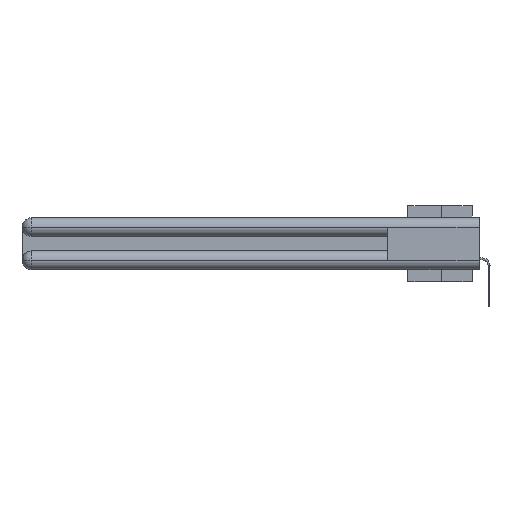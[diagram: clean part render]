
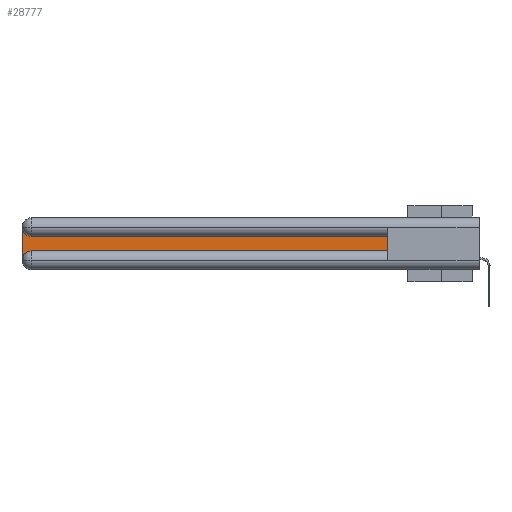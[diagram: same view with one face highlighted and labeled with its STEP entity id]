
A CAD part, left-side view. The second image highlights one B-rep face of the part: STEP entity #28777.
In plain terms, the highlighted planar face has unit normal (-1, 0, 0).
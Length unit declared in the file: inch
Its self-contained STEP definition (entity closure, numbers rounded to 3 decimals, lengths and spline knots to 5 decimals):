
#71 = DIRECTION ( 'NONE',  ( 0., 0., -1. ) ) ;
#74 = CARTESIAN_POINT ( 'NONE',  ( 0.075, 2.94, -0.2775 ) ) ;
#601 = AXIS2_PLACEMENT_3D ( 'NONE', #74, #2837, #3019 ) ;
#1091 = ORIENTED_EDGE ( 'NONE', *, *, #26982, .T. ) ;
#1092 = DIRECTION ( 'NONE',  ( 0., 0., -1. ) ) ;
#1126 = EDGE_CURVE ( 'NONE', #16371, #23580, #26672, .T. ) ;
#1837 = EDGE_CURVE ( 'NONE', #14054, #26302, #26580, .T. ) ;
#2837 = DIRECTION ( 'NONE',  ( 1., 0., 0. ) ) ;
#3019 = DIRECTION ( 'NONE',  ( 0., 0., -1. ) ) ;
#3077 = EDGE_CURVE ( 'NONE', #4866, #16371, #8599, .T. ) ;
#4682 = EDGE_CURVE ( 'NONE', #23580, #14054, #10926, .T. ) ;
#4866 = VERTEX_POINT ( 'NONE', #5899 ) ;
#5076 = CARTESIAN_POINT ( 'NONE',  ( 0.075, 0.6, -0.2175 ) ) ;
#5422 = FACE_OUTER_BOUND ( 'NONE', #32819, .T. ) ;
#5568 = CARTESIAN_POINT ( 'NONE',  ( 0.075, 2.94, -0.1225 ) ) ;
#5704 = CARTESIAN_POINT ( 'NONE',  ( 0.075, 2.94, -0.2175 ) ) ;
#5899 = CARTESIAN_POINT ( 'NONE',  ( 0.075, 0.6, -0.1225 ) ) ;
#6204 = LINE ( 'NONE', #17472, #26172 ) ;
#6418 = ORIENTED_EDGE ( 'NONE', *, *, #1126, .T. ) ;
#8599 = LINE ( 'NONE', #19509, #22413 ) ;
#9050 = CARTESIAN_POINT ( 'NONE',  ( 0.075, 2.94, -0.0625 ) ) ;
#10184 = ORIENTED_EDGE ( 'NONE', *, *, #4682, .T. ) ;
#10926 = LINE ( 'NONE', #16117, #13126 ) ;
#11690 = CARTESIAN_POINT ( 'NONE',  ( 0.075, 3., -0.1225 ) ) ;
#13126 = VECTOR ( 'NONE', #25139, 39.37008 ) ;
#13704 = AXIS2_PLACEMENT_3D ( 'NONE', #9050, #28813, #1092 ) ;
#13805 = DIRECTION ( 'NONE',  ( 0., 1., 0. ) ) ;
#14054 = VERTEX_POINT ( 'NONE', #29197 ) ;
#16117 = CARTESIAN_POINT ( 'NONE',  ( 0.075, 3., -0.2175 ) ) ;
#16333 = AXIS2_PLACEMENT_3D ( 'NONE', #11690, #30930, #71 ) ;
#16371 = VERTEX_POINT ( 'NONE', #5568 ) ;
#17219 = ORIENTED_EDGE ( 'NONE', *, *, #3077, .T. ) ;
#17472 = CARTESIAN_POINT ( 'NONE',  ( 0.075, 0.6, -0.2175 ) ) ;
#17829 = DIRECTION ( 'NONE',  ( 0., 0., 1. ) ) ;
#19509 = CARTESIAN_POINT ( 'NONE',  ( 0.075, 0.6, -0.1225 ) ) ;
#19995 = PLANE ( 'NONE',  #16333 ) ;
#22413 = VECTOR ( 'NONE', #13805, 39.37008 ) ;
#23580 = VERTEX_POINT ( 'NONE', #33311 ) ;
#24606 = VECTOR ( 'NONE', #24648, 39.37008 ) ;
#24648 = DIRECTION ( 'NONE',  ( 0., -1., 0. ) ) ;
#24835 = LINE ( 'NONE', #5076, #24606 ) ;
#25139 = DIRECTION ( 'NONE',  ( 0., 0., -1. ) ) ;
#26172 = VECTOR ( 'NONE', #17829, 39.37008 ) ;
#26302 = VERTEX_POINT ( 'NONE', #5704 ) ;
#26580 = CIRCLE ( 'NONE', #601, 0.06 ) ;
#26672 = CIRCLE ( 'NONE', #13704, 0.06 ) ;
#26982 = EDGE_CURVE ( 'NONE', #33030, #4866, #6204, .T. ) ;
#28777 = ADVANCED_FACE ( 'NONE', ( #5422 ), #19995, .F. ) ;
#28813 = DIRECTION ( 'NONE',  ( 1., 0., 0. ) ) ;
#29197 = CARTESIAN_POINT ( 'NONE',  ( 0.075, 3., -0.2775 ) ) ;
#29212 = ORIENTED_EDGE ( 'NONE', *, *, #1837, .T. ) ;
#30386 = EDGE_CURVE ( 'NONE', #26302, #33030, #24835, .T. ) ;
#30930 = DIRECTION ( 'NONE',  ( 1., 0., 0. ) ) ;
#31825 = ORIENTED_EDGE ( 'NONE', *, *, #30386, .T. ) ;
#32116 = CARTESIAN_POINT ( 'NONE',  ( 0.075, 0.6, -0.2175 ) ) ;
#32819 = EDGE_LOOP ( 'NONE', ( #17219, #6418, #10184, #29212, #31825, #1091 ) ) ;
#33030 = VERTEX_POINT ( 'NONE', #32116 ) ;
#33311 = CARTESIAN_POINT ( 'NONE',  ( 0.075, 3., -0.0625 ) ) ;
